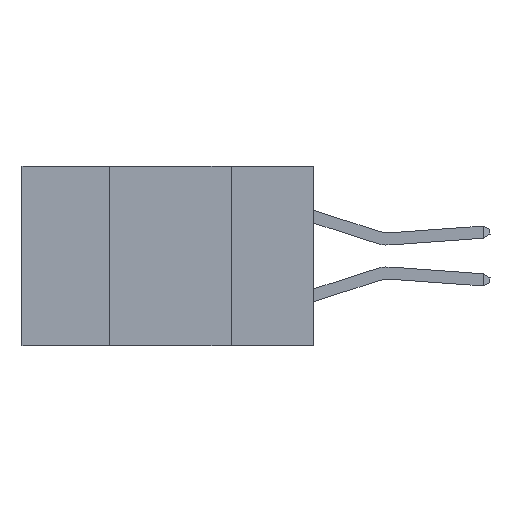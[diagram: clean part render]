
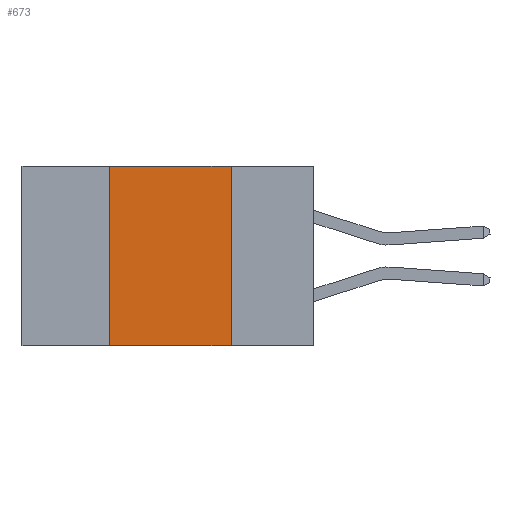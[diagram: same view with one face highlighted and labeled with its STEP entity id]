
A CAD part, left-side view. The second image highlights one B-rep face of the part: STEP entity #673.
In plain terms, the highlighted planar face has unit normal (-1, 0, 0).
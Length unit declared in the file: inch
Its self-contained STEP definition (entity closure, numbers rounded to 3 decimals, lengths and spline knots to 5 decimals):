
#639 = AXIS2_PLACEMENT_3D ( 'NONE', #9884, #13512, #14174 ) ;
#673 = ADVANCED_FACE ( 'NONE', ( #11920 ), #1323, .F. ) ;
#747 = CARTESIAN_POINT ( 'NONE',  ( 0., 0.6, 0. ) ) ;
#932 = ORIENTED_EDGE ( 'NONE', *, *, #7979, .F. ) ;
#1323 = PLANE ( 'NONE',  #639 ) ;
#1345 = DIRECTION ( 'NONE',  ( 0., 0., 1. ) ) ;
#1464 = CARTESIAN_POINT ( 'NONE',  ( 0., 0.6, -0.37 ) ) ;
#2127 = LINE ( 'NONE', #2618, #14966 ) ;
#2135 = DIRECTION ( 'NONE',  ( 0., -1., 0. ) ) ;
#2240 = VERTEX_POINT ( 'NONE', #6281 ) ;
#2618 = CARTESIAN_POINT ( 'NONE',  ( 0., 0.17, 0. ) ) ;
#4335 = ORIENTED_EDGE ( 'NONE', *, *, #15186, .F. ) ;
#4688 = VERTEX_POINT ( 'NONE', #13519 ) ;
#5600 = CARTESIAN_POINT ( 'NONE',  ( 0., 0.42, -0.37 ) ) ;
#6281 = CARTESIAN_POINT ( 'NONE',  ( 0., 0.17, 0. ) ) ;
#7294 = VECTOR ( 'NONE', #2135, 39.37008 ) ;
#7839 = CARTESIAN_POINT ( 'NONE',  ( 0., 0.42, 0. ) ) ;
#7979 = EDGE_CURVE ( 'NONE', #2240, #4688, #2127, .T. ) ;
#8438 = ORIENTED_EDGE ( 'NONE', *, *, #15234, .T. ) ;
#8540 = VECTOR ( 'NONE', #10367, 39.37008 ) ;
#9659 = VERTEX_POINT ( 'NONE', #13610 ) ;
#9884 = CARTESIAN_POINT ( 'NONE',  ( 0., 0.6, 0. ) ) ;
#10367 = DIRECTION ( 'NONE',  ( 0., -1., 0. ) ) ;
#11632 = EDGE_CURVE ( 'NONE', #9659, #2240, #13716, .T. ) ;
#11759 = EDGE_LOOP ( 'NONE', ( #932, #12606, #4335, #8438 ) ) ;
#11769 = VECTOR ( 'NONE', #1345, 39.37008 ) ;
#11920 = FACE_OUTER_BOUND ( 'NONE', #11759, .T. ) ;
#12064 = VERTEX_POINT ( 'NONE', #5600 ) ;
#12528 = LINE ( 'NONE', #7839, #11769 ) ;
#12606 = ORIENTED_EDGE ( 'NONE', *, *, #11632, .F. ) ;
#13512 = DIRECTION ( 'NONE',  ( 1., 0., 0. ) ) ;
#13519 = CARTESIAN_POINT ( 'NONE',  ( 0., 0.17, -0.37 ) ) ;
#13610 = CARTESIAN_POINT ( 'NONE',  ( 0., 0.42, 0. ) ) ;
#13716 = LINE ( 'NONE', #747, #7294 ) ;
#14174 = DIRECTION ( 'NONE',  ( 0., 0., -1. ) ) ;
#14586 = LINE ( 'NONE', #1464, #8540 ) ;
#14966 = VECTOR ( 'NONE', #15042, 39.37008 ) ;
#15042 = DIRECTION ( 'NONE',  ( 0., 0., -1. ) ) ;
#15186 = EDGE_CURVE ( 'NONE', #12064, #9659, #12528, .T. ) ;
#15234 = EDGE_CURVE ( 'NONE', #12064, #4688, #14586, .T. ) ;
